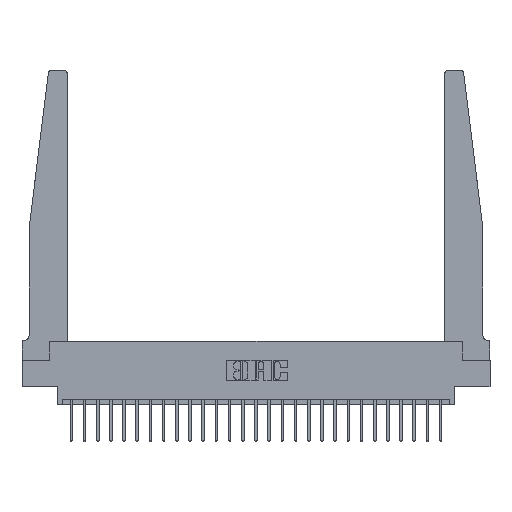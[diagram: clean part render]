
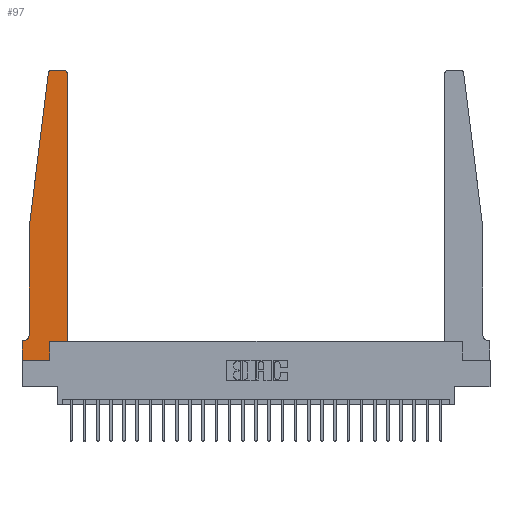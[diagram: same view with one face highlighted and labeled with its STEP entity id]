
A CAD part, top view. The second image highlights one B-rep face of the part: STEP entity #97.
In plain terms, the highlighted planar face has unit normal (0, 0, 1).
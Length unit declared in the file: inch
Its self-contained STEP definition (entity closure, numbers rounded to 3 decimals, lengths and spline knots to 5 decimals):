
#97 = ADVANCED_FACE ( 'NONE', ( #13514 ), #18816, .T. ) ;
#222 = AXIS2_PLACEMENT_3D ( 'NONE', #14056, #2220, #16072 ) ;
#265 = CARTESIAN_POINT ( 'NONE',  ( 0., 0., 0.37 ) ) ;
#844 = ORIENTED_EDGE ( 'NONE', *, *, #4683, .T. ) ;
#901 = DIRECTION ( 'NONE',  ( -1., 0., 0. ) ) ;
#907 = CARTESIAN_POINT ( 'NONE',  ( 0.065, 1.25, 0.37 ) ) ;
#931 = CARTESIAN_POINT ( 'NONE',  ( 0., 0., 0.37 ) ) ;
#1000 = CARTESIAN_POINT ( 'NONE',  ( 0.065, 1.25, 0.37 ) ) ;
#1060 = CARTESIAN_POINT ( 'NONE',  ( 0.065, 0.1875, 0.37 ) ) ;
#1190 = LINE ( 'NONE', #6551, #6460 ) ;
#1738 = DIRECTION ( 'NONE',  ( 0., 0., 1. ) ) ;
#1882 = VERTEX_POINT ( 'NONE', #1000 ) ;
#2220 = DIRECTION ( 'NONE',  ( 0., 0., -1. ) ) ;
#2270 = CARTESIAN_POINT ( 'NONE',  ( 0.2605, 0.18, 0.37 ) ) ;
#2435 = VECTOR ( 'NONE', #14735, 39.37008 ) ;
#2883 = CARTESIAN_POINT ( 'NONE',  ( 0.25, 2.75, 0.37 ) ) ;
#3398 = EDGE_CURVE ( 'NONE', #16473, #23308, #21129, .T. ) ;
#3696 = VECTOR ( 'NONE', #8996, 39.37008 ) ;
#3934 = ORIENTED_EDGE ( 'NONE', *, *, #25416, .T. ) ;
#4121 = CIRCLE ( 'NONE', #222, 0.05 ) ;
#4365 = VECTOR ( 'NONE', #8140, 39.37008 ) ;
#4459 = ORIENTED_EDGE ( 'NONE', *, *, #12274, .T. ) ;
#4485 = LINE ( 'NONE', #11335, #19657 ) ;
#4683 = EDGE_CURVE ( 'NONE', #20137, #1882, #10201, .T. ) ;
#4851 = VERTEX_POINT ( 'NONE', #21368 ) ;
#5270 = EDGE_CURVE ( 'NONE', #1882, #22589, #7103, .T. ) ;
#5689 = ORIENTED_EDGE ( 'NONE', *, *, #5270, .T. ) ;
#6153 = EDGE_CURVE ( 'NONE', #23113, #6783, #24755, .T. ) ;
#6460 = VECTOR ( 'NONE', #8523, 39.37008 ) ;
#6551 = CARTESIAN_POINT ( 'NONE',  ( 0., 0., 0.37 ) ) ;
#6649 = VERTEX_POINT ( 'NONE', #22267 ) ;
#6783 = VERTEX_POINT ( 'NONE', #8834 ) ;
#6982 = CARTESIAN_POINT ( 'NONE',  ( 0., 0.1875, 0.37 ) ) ;
#7103 = LINE ( 'NONE', #907, #2435 ) ;
#7189 = ORIENTED_EDGE ( 'NONE', *, *, #12717, .T. ) ;
#7329 = ORIENTED_EDGE ( 'NONE', *, *, #21002, .T. ) ;
#8016 = CARTESIAN_POINT ( 'NONE',  ( 0.395, 2.72, 0.37 ) ) ;
#8041 = EDGE_CURVE ( 'NONE', #23039, #4851, #19722, .T. ) ;
#8140 = DIRECTION ( 'NONE',  ( 1., 0., 0. ) ) ;
#8214 = CARTESIAN_POINT ( 'NONE',  ( 0.395, 2.75, 0.37 ) ) ;
#8523 = DIRECTION ( 'NONE',  ( 0., -1., 0. ) ) ;
#8727 = CIRCLE ( 'NONE', #9497, 0.03 ) ;
#8834 = CARTESIAN_POINT ( 'NONE',  ( 0., 0.1875, 0.37 ) ) ;
#8955 = VECTOR ( 'NONE', #24883, 39.37008 ) ;
#8969 = DIRECTION ( 'NONE',  ( 0., 0., 1. ) ) ;
#8996 = DIRECTION ( 'NONE',  ( -0.122, -0.992, 0. ) ) ;
#9497 = AXIS2_PLACEMENT_3D ( 'NONE', #13575, #1738, #15577 ) ;
#9681 = ORIENTED_EDGE ( 'NONE', *, *, #6153, .T. ) ;
#10004 = DIRECTION ( 'NONE',  ( 1., 0., 0. ) ) ;
#10172 = CIRCLE ( 'NONE', #15562, 0.03 ) ;
#10201 = LINE ( 'NONE', #18847, #3696 ) ;
#10401 = CARTESIAN_POINT ( 'NONE',  ( 0.2605, 0.18, 0.37 ) ) ;
#10988 = ORIENTED_EDGE ( 'NONE', *, *, #25231, .T. ) ;
#11335 = CARTESIAN_POINT ( 'NONE',  ( 0.425, 0.18, 0.37 ) ) ;
#11428 = DIRECTION ( 'NONE',  ( 0., 1., 0. ) ) ;
#11455 = VECTOR ( 'NONE', #12195, 39.37008 ) ;
#12195 = DIRECTION ( 'NONE',  ( 0., 1., 0. ) ) ;
#12274 = EDGE_CURVE ( 'NONE', #6649, #23039, #22012, .T. ) ;
#12717 = EDGE_CURVE ( 'NONE', #4851, #17266, #4485, .T. ) ;
#13461 = EDGE_CURVE ( 'NONE', #22589, #23113, #4121, .T. ) ;
#13514 = FACE_OUTER_BOUND ( 'NONE', #18944, .T. ) ;
#13575 = CARTESIAN_POINT ( 'NONE',  ( 0.27653, 2.72, 0.37 ) ) ;
#14056 = CARTESIAN_POINT ( 'NONE',  ( 0.015, 0.2375, 0.37 ) ) ;
#14448 = VECTOR ( 'NONE', #14643, 39.37008 ) ;
#14643 = DIRECTION ( 'NONE',  ( 1., 0., 0. ) ) ;
#14735 = DIRECTION ( 'NONE',  ( 0., -1., 0. ) ) ;
#15168 = ORIENTED_EDGE ( 'NONE', *, *, #20808, .T. ) ;
#15515 = LINE ( 'NONE', #265, #4365 ) ;
#15562 = AXIS2_PLACEMENT_3D ( 'NONE', #8016, #21883, #10004 ) ;
#15577 = DIRECTION ( 'NONE',  ( 1., 0., 0. ) ) ;
#15703 = CARTESIAN_POINT ( 'NONE',  ( 0.065, 0.2375, 0.37 ) ) ;
#16072 = DIRECTION ( 'NONE',  ( -1., 0., 0. ) ) ;
#16473 = VERTEX_POINT ( 'NONE', #8214 ) ;
#16563 = CARTESIAN_POINT ( 'NONE',  ( 0.425, 2.72, 0.37 ) ) ;
#16633 = CARTESIAN_POINT ( 'NONE',  ( 0.425, 0.18, 0.37 ) ) ;
#17266 = VERTEX_POINT ( 'NONE', #16563 ) ;
#18751 = VERTEX_POINT ( 'NONE', #931 ) ;
#18816 = PLANE ( 'NONE',  #25581 ) ;
#18847 = CARTESIAN_POINT ( 'NONE',  ( 0.065, 1.25, 0.37 ) ) ;
#18944 = EDGE_LOOP ( 'NONE', ( #19795, #10988, #844, #5689, #24761, #9681, #7329, #3934, #4459, #24411, #7189, #15168 ) ) ;
#19572 = CARTESIAN_POINT ( 'NONE',  ( 0.27653, 2.75, 0.37 ) ) ;
#19657 = VECTOR ( 'NONE', #11428, 39.37008 ) ;
#19722 = LINE ( 'NONE', #16633, #14448 ) ;
#19795 = ORIENTED_EDGE ( 'NONE', *, *, #3398, .T. ) ;
#20137 = VERTEX_POINT ( 'NONE', #21645 ) ;
#20464 = CARTESIAN_POINT ( 'NONE',  ( 0.015, 0.1875, 0.37 ) ) ;
#20511 = VECTOR ( 'NONE', #901, 39.37008 ) ;
#20808 = EDGE_CURVE ( 'NONE', #17266, #16473, #10172, .T. ) ;
#21002 = EDGE_CURVE ( 'NONE', #6783, #18751, #1190, .T. ) ;
#21129 = LINE ( 'NONE', #2883, #20511 ) ;
#21368 = CARTESIAN_POINT ( 'NONE',  ( 0.425, 0.18, 0.37 ) ) ;
#21645 = CARTESIAN_POINT ( 'NONE',  ( 0.24675, 2.72367, 0.37 ) ) ;
#21883 = DIRECTION ( 'NONE',  ( 0., 0., 1. ) ) ;
#22012 = LINE ( 'NONE', #2270, #11455 ) ;
#22267 = CARTESIAN_POINT ( 'NONE',  ( 0.2605, 0., 0.37 ) ) ;
#22589 = VERTEX_POINT ( 'NONE', #15703 ) ;
#22839 = DIRECTION ( 'NONE',  ( 1., 0., 0. ) ) ;
#23039 = VERTEX_POINT ( 'NONE', #10401 ) ;
#23113 = VERTEX_POINT ( 'NONE', #20464 ) ;
#23308 = VERTEX_POINT ( 'NONE', #19572 ) ;
#24411 = ORIENTED_EDGE ( 'NONE', *, *, #8041, .T. ) ;
#24755 = LINE ( 'NONE', #1060, #8955 ) ;
#24761 = ORIENTED_EDGE ( 'NONE', *, *, #13461, .T. ) ;
#24883 = DIRECTION ( 'NONE',  ( -1., 0., 0. ) ) ;
#25231 = EDGE_CURVE ( 'NONE', #23308, #20137, #8727, .T. ) ;
#25416 = EDGE_CURVE ( 'NONE', #18751, #6649, #15515, .T. ) ;
#25581 = AXIS2_PLACEMENT_3D ( 'NONE', #6982, #8969, #22839 ) ;
